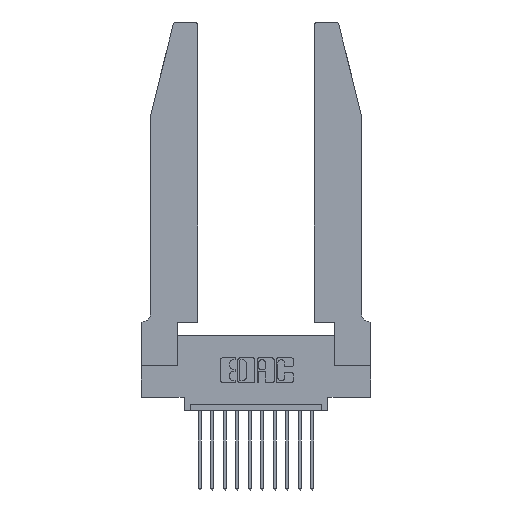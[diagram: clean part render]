
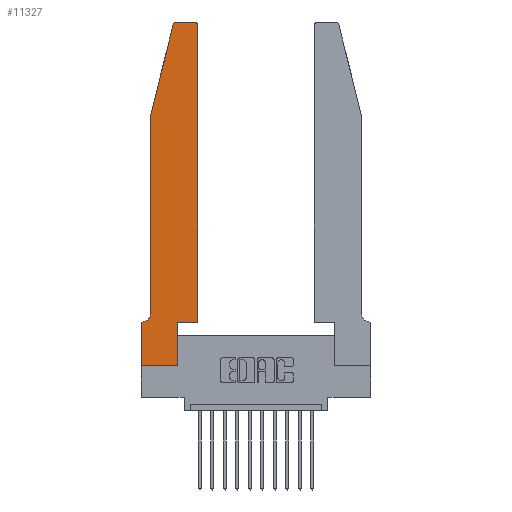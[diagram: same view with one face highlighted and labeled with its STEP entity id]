
A CAD part, top view. The second image highlights one B-rep face of the part: STEP entity #11327.
In plain terms, the highlighted planar face has unit normal (0, 0, 1).
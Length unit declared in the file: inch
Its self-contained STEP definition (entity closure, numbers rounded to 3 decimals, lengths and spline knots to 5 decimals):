
#84 = EDGE_CURVE ( 'NONE', #5358, #2693, #3838, .T. ) ;
#121 = ORIENTED_EDGE ( 'NONE', *, *, #1551, .T. ) ;
#155 = CARTESIAN_POINT ( 'NONE',  ( 0.4505, 0.35, 0.37 ) ) ;
#489 = VECTOR ( 'NONE', #2968, 39.37008 ) ;
#565 = VECTOR ( 'NONE', #2539, 39.37008 ) ;
#728 = DIRECTION ( 'NONE',  ( -1., 0., 0. ) ) ;
#733 = LINE ( 'NONE', #155, #12494 ) ;
#760 = LINE ( 'NONE', #6999, #5869 ) ;
#790 = VERTEX_POINT ( 'NONE', #11418 ) ;
#793 = ORIENTED_EDGE ( 'NONE', *, *, #3099, .T. ) ;
#954 = EDGE_CURVE ( 'NONE', #2517, #3878, #3965, .T. ) ;
#1016 = ORIENTED_EDGE ( 'NONE', *, *, #10311, .T. ) ;
#1211 = DIRECTION ( 'NONE',  ( 1., 0., 0. ) ) ;
#1227 = DIRECTION ( 'NONE',  ( 0., 0., 1. ) ) ;
#1497 = CIRCLE ( 'NONE', #11514, 0.03 ) ;
#1499 = DIRECTION ( 'NONE',  ( 0., -1., 0. ) ) ;
#1551 = EDGE_CURVE ( 'NONE', #2693, #14456, #733, .T. ) ;
#1756 = CARTESIAN_POINT ( 'NONE',  ( 0.4205, 2.75, 0.37 ) ) ;
#2347 = DIRECTION ( 'NONE',  ( 0., 0., 1. ) ) ;
#2397 = VECTOR ( 'NONE', #728, 39.37008 ) ;
#2517 = VERTEX_POINT ( 'NONE', #13974 ) ;
#2539 = DIRECTION ( 'NONE',  ( 0., -1., 0. ) ) ;
#2590 = LINE ( 'NONE', #11308, #5678 ) ;
#2693 = VERTEX_POINT ( 'NONE', #13609 ) ;
#2705 = DIRECTION ( 'NONE',  ( 0., 1., 0. ) ) ;
#2767 = VERTEX_POINT ( 'NONE', #12384 ) ;
#2901 = ORIENTED_EDGE ( 'NONE', *, *, #3195, .T. ) ;
#2961 = CARTESIAN_POINT ( 'NONE',  ( 0.2865, 0., 0.37 ) ) ;
#2968 = DIRECTION ( 'NONE',  ( 0., 1., 0. ) ) ;
#3099 = EDGE_CURVE ( 'NONE', #2767, #16631, #1497, .T. ) ;
#3120 = EDGE_CURVE ( 'NONE', #16631, #4177, #10479, .T. ) ;
#3195 = EDGE_CURVE ( 'NONE', #8495, #2517, #4537, .T. ) ;
#3703 = CARTESIAN_POINT ( 'NONE',  ( 0.284, 2.75, 0.37 ) ) ;
#3766 = CARTESIAN_POINT ( 'NONE',  ( 0.0755, 2., 0.37 ) ) ;
#3838 = LINE ( 'NONE', #13244, #5531 ) ;
#3877 = ORIENTED_EDGE ( 'NONE', *, *, #11035, .T. ) ;
#3878 = VERTEX_POINT ( 'NONE', #13311 ) ;
#3965 = LINE ( 'NONE', #3766, #565 ) ;
#3999 = CARTESIAN_POINT ( 'NONE',  ( 0.0055, 0.42, 0.37 ) ) ;
#4177 = VERTEX_POINT ( 'NONE', #3703 ) ;
#4537 = LINE ( 'NONE', #15899, #13671 ) ;
#5070 = EDGE_CURVE ( 'NONE', #4177, #8495, #9989, .T. ) ;
#5217 = CARTESIAN_POINT ( 'NONE',  ( 0., 0., 0.37 ) ) ;
#5351 = CARTESIAN_POINT ( 'NONE',  ( 0.4205, 2.72, 0.37 ) ) ;
#5358 = VERTEX_POINT ( 'NONE', #2961 ) ;
#5365 = DIRECTION ( 'NONE',  ( 0., 0., -1. ) ) ;
#5531 = VECTOR ( 'NONE', #2705, 39.37008 ) ;
#5678 = VECTOR ( 'NONE', #16471, 39.37008 ) ;
#5869 = VECTOR ( 'NONE', #1499, 39.37008 ) ;
#6186 = LINE ( 'NONE', #12210, #489 ) ;
#6826 = AXIS2_PLACEMENT_3D ( 'NONE', #3999, #5365, #9406 ) ;
#6999 = CARTESIAN_POINT ( 'NONE',  ( 0., 0., 0.37 ) ) ;
#7181 = EDGE_CURVE ( 'NONE', #11320, #13145, #760, .T. ) ;
#7540 = EDGE_CURVE ( 'NONE', #14456, #2767, #6186, .T. ) ;
#7571 = CARTESIAN_POINT ( 'NONE',  ( 0., 0.35, 0.37 ) ) ;
#7680 = CARTESIAN_POINT ( 'NONE',  ( 0., 0.35, 0.37 ) ) ;
#7699 = LINE ( 'NONE', #16446, #2397 ) ;
#8076 = DIRECTION ( 'NONE',  ( -0.239, -0.971, 0. ) ) ;
#8495 = VERTEX_POINT ( 'NONE', #9986 ) ;
#8878 = PLANE ( 'NONE',  #14824 ) ;
#9244 = ORIENTED_EDGE ( 'NONE', *, *, #10591, .T. ) ;
#9406 = DIRECTION ( 'NONE',  ( -1., 0., 0. ) ) ;
#9768 = ORIENTED_EDGE ( 'NONE', *, *, #84, .T. ) ;
#9839 = ORIENTED_EDGE ( 'NONE', *, *, #5070, .T. ) ;
#9986 = CARTESIAN_POINT ( 'NONE',  ( 0.25487, 2.72718, 0.37 ) ) ;
#9989 = CIRCLE ( 'NONE', #11628, 0.03 ) ;
#10156 = CARTESIAN_POINT ( 'NONE',  ( 0.284, 2.72, 0.37 ) ) ;
#10311 = EDGE_CURVE ( 'NONE', #3878, #790, #15975, .T. ) ;
#10479 = LINE ( 'NONE', #11920, #14487 ) ;
#10591 = EDGE_CURVE ( 'NONE', #790, #11320, #7699, .T. ) ;
#10637 = DIRECTION ( 'NONE',  ( 1., 0., 0. ) ) ;
#11035 = EDGE_CURVE ( 'NONE', #13145, #5358, #2590, .T. ) ;
#11308 = CARTESIAN_POINT ( 'NONE',  ( 0., 0., 0.37 ) ) ;
#11320 = VERTEX_POINT ( 'NONE', #7571 ) ;
#11327 = ADVANCED_FACE ( 'NONE', ( #15949 ), #8878, .T. ) ;
#11418 = CARTESIAN_POINT ( 'NONE',  ( 0.0055, 0.35, 0.37 ) ) ;
#11514 = AXIS2_PLACEMENT_3D ( 'NONE', #5351, #11866, #10637 ) ;
#11628 = AXIS2_PLACEMENT_3D ( 'NONE', #10156, #2347, #16652 ) ;
#11866 = DIRECTION ( 'NONE',  ( 0., 0., 1. ) ) ;
#11920 = CARTESIAN_POINT ( 'NONE',  ( 0.2605, 2.75, 0.37 ) ) ;
#12115 = ORIENTED_EDGE ( 'NONE', *, *, #954, .T. ) ;
#12210 = CARTESIAN_POINT ( 'NONE',  ( 0.4505, 0.35, 0.37 ) ) ;
#12384 = CARTESIAN_POINT ( 'NONE',  ( 0.4505, 2.72, 0.37 ) ) ;
#12494 = VECTOR ( 'NONE', #1211, 39.37008 ) ;
#12791 = DIRECTION ( 'NONE',  ( 1., 0., 0. ) ) ;
#13145 = VERTEX_POINT ( 'NONE', #5217 ) ;
#13244 = CARTESIAN_POINT ( 'NONE',  ( 0.2865, 0.35, 0.37 ) ) ;
#13311 = CARTESIAN_POINT ( 'NONE',  ( 0.0755, 0.42, 0.37 ) ) ;
#13598 = ORIENTED_EDGE ( 'NONE', *, *, #3120, .T. ) ;
#13609 = CARTESIAN_POINT ( 'NONE',  ( 0.2865, 0.35, 0.37 ) ) ;
#13671 = VECTOR ( 'NONE', #8076, 39.37008 ) ;
#13974 = CARTESIAN_POINT ( 'NONE',  ( 0.0755, 2., 0.37 ) ) ;
#14279 = CARTESIAN_POINT ( 'NONE',  ( 0.4505, 0.35, 0.37 ) ) ;
#14398 = DIRECTION ( 'NONE',  ( -1., 0., 0. ) ) ;
#14456 = VERTEX_POINT ( 'NONE', #14279 ) ;
#14487 = VECTOR ( 'NONE', #14398, 39.37008 ) ;
#14824 = AXIS2_PLACEMENT_3D ( 'NONE', #7680, #1227, #12791 ) ;
#15147 = ORIENTED_EDGE ( 'NONE', *, *, #7181, .T. ) ;
#15246 = EDGE_LOOP ( 'NONE', ( #13598, #9839, #2901, #12115, #1016, #9244, #15147, #3877, #9768, #121, #16608, #793 ) ) ;
#15899 = CARTESIAN_POINT ( 'NONE',  ( 0.0755, 2., 0.37 ) ) ;
#15949 = FACE_OUTER_BOUND ( 'NONE', #15246, .T. ) ;
#15975 = CIRCLE ( 'NONE', #6826, 0.07 ) ;
#16446 = CARTESIAN_POINT ( 'NONE',  ( 0.0755, 0.35, 0.37 ) ) ;
#16471 = DIRECTION ( 'NONE',  ( 1., 0., 0. ) ) ;
#16608 = ORIENTED_EDGE ( 'NONE', *, *, #7540, .T. ) ;
#16631 = VERTEX_POINT ( 'NONE', #1756 ) ;
#16652 = DIRECTION ( 'NONE',  ( 1., 0., 0. ) ) ;
